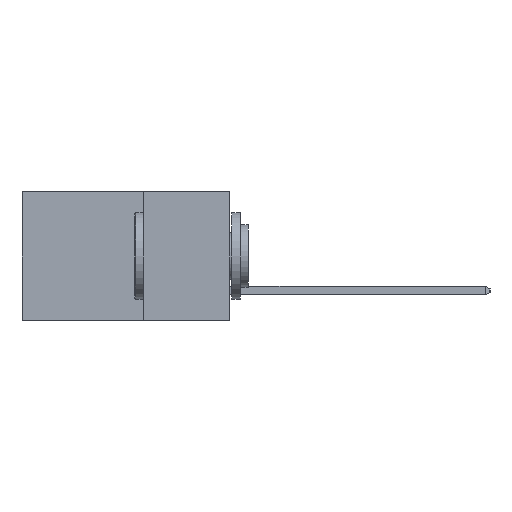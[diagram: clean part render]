
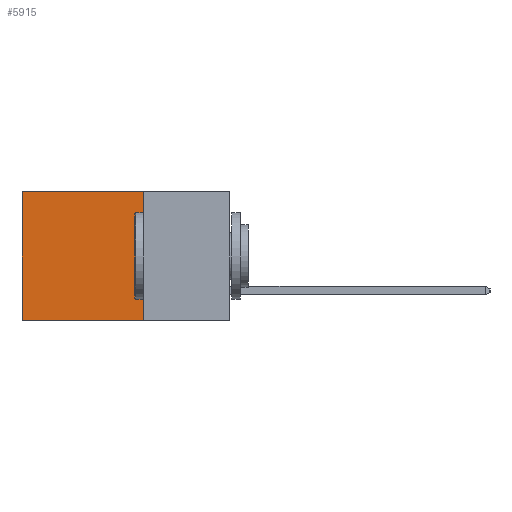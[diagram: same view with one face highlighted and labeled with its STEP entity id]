
A CAD part, left-side view. The second image highlights one B-rep face of the part: STEP entity #5915.
In plain terms, the highlighted planar face has unit normal (-1, 0, 0).
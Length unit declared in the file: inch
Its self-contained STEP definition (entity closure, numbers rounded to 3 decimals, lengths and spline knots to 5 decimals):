
#442 = ORIENTED_EDGE ( 'NONE', *, *, #10588, .T. ) ;
#507 = VERTEX_POINT ( 'NONE', #8346 ) ;
#2604 = CARTESIAN_POINT ( 'NONE',  ( 0.2615, 0.6, 0. ) ) ;
#3172 = EDGE_CURVE ( 'NONE', #8208, #507, #16675, .T. ) ;
#3487 = EDGE_LOOP ( 'NONE', ( #12354, #13588, #20741, #442 ) ) ;
#3946 = DIRECTION ( 'NONE',  ( 0., 1., 0. ) ) ;
#4282 = CARTESIAN_POINT ( 'NONE',  ( 0.2615, 0.25, -0.37 ) ) ;
#5915 = ADVANCED_FACE ( 'NONE', ( #16334 ), #17459, .F. ) ;
#6249 = VECTOR ( 'NONE', #16301, 39.37008 ) ;
#7683 = DIRECTION ( 'NONE',  ( 1., 0., 0. ) ) ;
#7717 = VERTEX_POINT ( 'NONE', #2604 ) ;
#8208 = VERTEX_POINT ( 'NONE', #16330 ) ;
#8346 = CARTESIAN_POINT ( 'NONE',  ( 0.2615, 0.6, -0.37 ) ) ;
#8659 = AXIS2_PLACEMENT_3D ( 'NONE', #20007, #7683, #18040 ) ;
#8683 = VECTOR ( 'NONE', #9650, 39.37008 ) ;
#9026 = CARTESIAN_POINT ( 'NONE',  ( 0.2615, 0.6, -0.37 ) ) ;
#9167 = LINE ( 'NONE', #9421, #17444 ) ;
#9342 = DIRECTION ( 'NONE',  ( 0., 0., -1. ) ) ;
#9421 = CARTESIAN_POINT ( 'NONE',  ( 0.2615, 0.25, -0.37 ) ) ;
#9650 = DIRECTION ( 'NONE',  ( 0., 0., -1. ) ) ;
#10588 = EDGE_CURVE ( 'NONE', #15404, #7717, #15203, .T. ) ;
#12354 = ORIENTED_EDGE ( 'NONE', *, *, #14695, .T. ) ;
#13588 = ORIENTED_EDGE ( 'NONE', *, *, #3172, .F. ) ;
#14695 = EDGE_CURVE ( 'NONE', #7717, #507, #18993, .T. ) ;
#15203 = LINE ( 'NONE', #16265, #6249 ) ;
#15404 = VERTEX_POINT ( 'NONE', #19537 ) ;
#16000 = EDGE_CURVE ( 'NONE', #15404, #8208, #9167, .T. ) ;
#16167 = VECTOR ( 'NONE', #3946, 39.37008 ) ;
#16265 = CARTESIAN_POINT ( 'NONE',  ( 0.2615, 0.25, 0. ) ) ;
#16301 = DIRECTION ( 'NONE',  ( 0., 1., 0. ) ) ;
#16330 = CARTESIAN_POINT ( 'NONE',  ( 0.2615, 0.25, -0.37 ) ) ;
#16334 = FACE_OUTER_BOUND ( 'NONE', #3487, .T. ) ;
#16675 = LINE ( 'NONE', #4282, #16167 ) ;
#17444 = VECTOR ( 'NONE', #9342, 39.37008 ) ;
#17459 = PLANE ( 'NONE',  #8659 ) ;
#18040 = DIRECTION ( 'NONE',  ( 0., 0., -1. ) ) ;
#18993 = LINE ( 'NONE', #9026, #8683 ) ;
#19537 = CARTESIAN_POINT ( 'NONE',  ( 0.2615, 0.25, 0. ) ) ;
#20007 = CARTESIAN_POINT ( 'NONE',  ( 0.2615, 0.25, -0.37 ) ) ;
#20741 = ORIENTED_EDGE ( 'NONE', *, *, #16000, .F. ) ;
